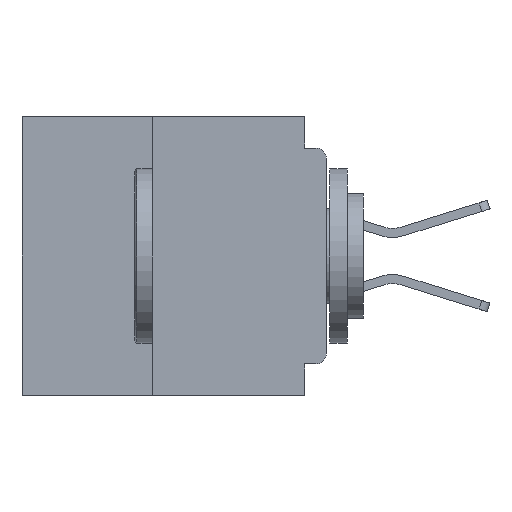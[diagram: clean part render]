
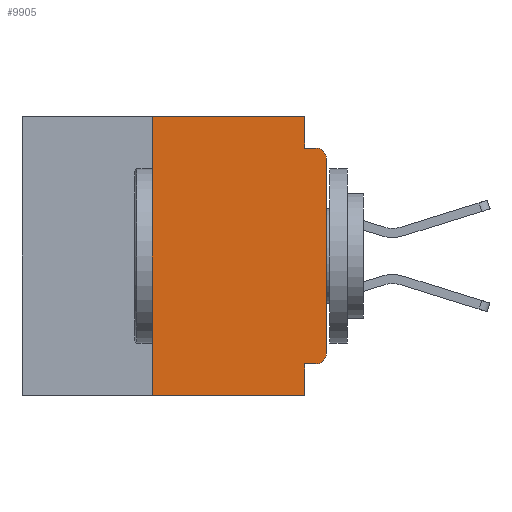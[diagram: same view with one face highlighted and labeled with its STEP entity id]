
A CAD part, left-side view. The second image highlights one B-rep face of the part: STEP entity #9905.
In plain terms, the highlighted planar face has unit normal (-1, 0, 0).
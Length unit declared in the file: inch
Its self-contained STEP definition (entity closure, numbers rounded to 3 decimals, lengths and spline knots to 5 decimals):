
#12 = CARTESIAN_POINT ( 'NONE',  ( 0., 0., -0.045 ) ) ;
#208 = VECTOR ( 'NONE', #36433, 39.37008 ) ;
#2026 = CARTESIAN_POINT ( 'NONE',  ( 0., 0.015, -0.045 ) ) ;
#2137 = DIRECTION ( 'NONE',  ( 0., 0., 1. ) ) ;
#2525 = EDGE_CURVE ( 'NONE', #13871, #28414, #29229, .T. ) ;
#3291 = DIRECTION ( 'NONE',  ( 0., 0., -1. ) ) ;
#3432 = DIRECTION ( 'NONE',  ( 0., -1., 0. ) ) ;
#4204 = CARTESIAN_POINT ( 'NONE',  ( 0., 0.437, 0. ) ) ;
#4430 = VERTEX_POINT ( 'NONE', #6940 ) ;
#4449 = ORIENTED_EDGE ( 'NONE', *, *, #25047, .F. ) ;
#4616 = ORIENTED_EDGE ( 'NONE', *, *, #38706, .F. ) ;
#5484 = DIRECTION ( 'NONE',  ( 0., -1., 0. ) ) ;
#5835 = FACE_OUTER_BOUND ( 'NONE', #27483, .T. ) ;
#6090 = AXIS2_PLACEMENT_3D ( 'NONE', #4204, #27766, #7579 ) ;
#6940 = CARTESIAN_POINT ( 'NONE',  ( 0., 0.031, 0. ) ) ;
#7013 = DIRECTION ( 'NONE',  ( 0., -1., 0. ) ) ;
#7579 = DIRECTION ( 'NONE',  ( 0., 0., -1. ) ) ;
#7852 = EDGE_CURVE ( 'NONE', #24211, #28414, #11741, .T. ) ;
#8002 = VERTEX_POINT ( 'NONE', #17994 ) ;
#8497 = VECTOR ( 'NONE', #5484, 39.37008 ) ;
#8793 = VERTEX_POINT ( 'NONE', #2026 ) ;
#8879 = CARTESIAN_POINT ( 'NONE',  ( 0., 0.031, -0.4 ) ) ;
#9077 = VECTOR ( 'NONE', #32143, 39.37008 ) ;
#9132 = DIRECTION ( 'NONE',  ( 0., 0., -1. ) ) ;
#9160 = CARTESIAN_POINT ( 'NONE',  ( 0., 0.031, -0.355 ) ) ;
#9869 = DIRECTION ( 'NONE',  ( 0., 0., 1. ) ) ;
#9905 = ADVANCED_FACE ( 'NONE', ( #5835 ), #37666, .F. ) ;
#9953 = CARTESIAN_POINT ( 'NONE',  ( 0., 0.25, -0.4 ) ) ;
#10318 = DIRECTION ( 'NONE',  ( -1., 0., 0. ) ) ;
#11296 = LINE ( 'NONE', #23139, #208 ) ;
#11741 = LINE ( 'NONE', #13603, #29705 ) ;
#12203 = LINE ( 'NONE', #28794, #9077 ) ;
#12559 = ORIENTED_EDGE ( 'NONE', *, *, #7852, .T. ) ;
#13377 = EDGE_CURVE ( 'NONE', #18714, #27841, #27173, .T. ) ;
#13603 = CARTESIAN_POINT ( 'NONE',  ( 0., 0.437, -0.4 ) ) ;
#13871 = VERTEX_POINT ( 'NONE', #9160 ) ;
#14904 = LINE ( 'NONE', #33392, #32845 ) ;
#14933 = CARTESIAN_POINT ( 'NONE',  ( 0., 0.031, -0.4 ) ) ;
#15539 = CARTESIAN_POINT ( 'NONE',  ( 0., 0.25, -0.4 ) ) ;
#16541 = EDGE_CURVE ( 'NONE', #27841, #41933, #14904, .T. ) ;
#16649 = CIRCLE ( 'NONE', #20965, 0.015 ) ;
#17417 = LINE ( 'NONE', #22259, #8497 ) ;
#17994 = CARTESIAN_POINT ( 'NONE',  ( 0., 0.031, -0.045 ) ) ;
#18585 = VECTOR ( 'NONE', #2137, 39.37008 ) ;
#18714 = VERTEX_POINT ( 'NONE', #41886 ) ;
#20965 = AXIS2_PLACEMENT_3D ( 'NONE', #30503, #10318, #33837 ) ;
#21598 = EDGE_CURVE ( 'NONE', #4430, #8002, #11296, .T. ) ;
#21882 = VECTOR ( 'NONE', #3432, 39.37008 ) ;
#22259 = CARTESIAN_POINT ( 'NONE',  ( 0., 0.437, 0. ) ) ;
#22960 = LINE ( 'NONE', #12, #21882 ) ;
#23139 = CARTESIAN_POINT ( 'NONE',  ( 0., 0.031, 0. ) ) ;
#23491 = DIRECTION ( 'NONE',  ( -1., 0., 0. ) ) ;
#24211 = VERTEX_POINT ( 'NONE', #9953 ) ;
#24551 = ORIENTED_EDGE ( 'NONE', *, *, #29446, .T. ) ;
#25047 = EDGE_CURVE ( 'NONE', #18714, #13871, #12203, .T. ) ;
#26115 = ORIENTED_EDGE ( 'NONE', *, *, #13377, .T. ) ;
#27173 = CIRCLE ( 'NONE', #30689, 0.015 ) ;
#27483 = EDGE_LOOP ( 'NONE', ( #29576, #24551, #33704, #38954, #33650, #4616, #12559, #41719, #4449, #26115 ) ) ;
#27605 = LINE ( 'NONE', #15539, #18585 ) ;
#27766 = DIRECTION ( 'NONE',  ( 1., 0., 0. ) ) ;
#27841 = VERTEX_POINT ( 'NONE', #35559 ) ;
#28414 = VERTEX_POINT ( 'NONE', #14933 ) ;
#28794 = CARTESIAN_POINT ( 'NONE',  ( 0., 0., -0.355 ) ) ;
#29229 = LINE ( 'NONE', #8879, #38047 ) ;
#29446 = EDGE_CURVE ( 'NONE', #41933, #8793, #16649, .T. ) ;
#29539 = CARTESIAN_POINT ( 'NONE',  ( 0., 0.25, 0. ) ) ;
#29576 = ORIENTED_EDGE ( 'NONE', *, *, #16541, .T. ) ;
#29705 = VECTOR ( 'NONE', #7013, 39.37008 ) ;
#30503 = CARTESIAN_POINT ( 'NONE',  ( 0., 0.015, -0.06 ) ) ;
#30689 = AXIS2_PLACEMENT_3D ( 'NONE', #43385, #23491, #3291 ) ;
#32085 = VERTEX_POINT ( 'NONE', #29539 ) ;
#32143 = DIRECTION ( 'NONE',  ( 0., 1., 0. ) ) ;
#32845 = VECTOR ( 'NONE', #9869, 39.37008 ) ;
#33392 = CARTESIAN_POINT ( 'NONE',  ( 0., 0., 0. ) ) ;
#33650 = ORIENTED_EDGE ( 'NONE', *, *, #40040, .F. ) ;
#33704 = ORIENTED_EDGE ( 'NONE', *, *, #41513, .F. ) ;
#33837 = DIRECTION ( 'NONE',  ( 0., 0., -1. ) ) ;
#35559 = CARTESIAN_POINT ( 'NONE',  ( 0., 0., -0.34 ) ) ;
#36433 = DIRECTION ( 'NONE',  ( 0., 0., -1. ) ) ;
#37666 = PLANE ( 'NONE',  #6090 ) ;
#38047 = VECTOR ( 'NONE', #9132, 39.37008 ) ;
#38706 = EDGE_CURVE ( 'NONE', #24211, #32085, #27605, .T. ) ;
#38954 = ORIENTED_EDGE ( 'NONE', *, *, #21598, .F. ) ;
#40040 = EDGE_CURVE ( 'NONE', #32085, #4430, #17417, .T. ) ;
#41513 = EDGE_CURVE ( 'NONE', #8002, #8793, #22960, .T. ) ;
#41719 = ORIENTED_EDGE ( 'NONE', *, *, #2525, .F. ) ;
#41886 = CARTESIAN_POINT ( 'NONE',  ( 0., 0.015, -0.355 ) ) ;
#41933 = VERTEX_POINT ( 'NONE', #42943 ) ;
#42943 = CARTESIAN_POINT ( 'NONE',  ( 0., 0., -0.06 ) ) ;
#43385 = CARTESIAN_POINT ( 'NONE',  ( 0., 0.015, -0.34 ) ) ;
